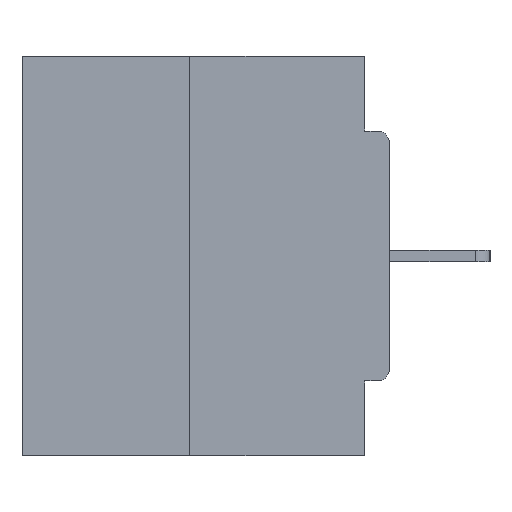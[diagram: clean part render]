
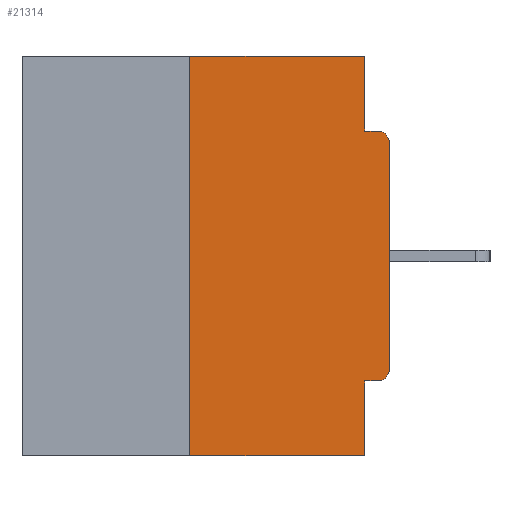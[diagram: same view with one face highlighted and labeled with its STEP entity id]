
A CAD part, left-side view. The second image highlights one B-rep face of the part: STEP entity #21314.
In plain terms, the highlighted planar face has unit normal (-1, 0, 0).
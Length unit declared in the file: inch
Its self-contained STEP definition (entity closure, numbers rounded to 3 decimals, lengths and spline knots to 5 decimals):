
#153 = VERTEX_POINT ( 'NONE', #30032 ) ;
#225 = LINE ( 'NONE', #2514, #6856 ) ;
#601 = EDGE_CURVE ( 'NONE', #12943, #153, #3066, .T. ) ;
#760 = EDGE_CURVE ( 'NONE', #32291, #30351, #11980, .T. ) ;
#1332 = CARTESIAN_POINT ( 'NONE',  ( 0., 0.031, -0.4065 ) ) ;
#1502 = CARTESIAN_POINT ( 'NONE',  ( 0., 0., -0.1085 ) ) ;
#1536 = LINE ( 'NONE', #28519, #22157 ) ;
#2011 = FACE_OUTER_BOUND ( 'NONE', #24314, .T. ) ;
#2514 = CARTESIAN_POINT ( 'NONE',  ( 0., 0., -0.4065 ) ) ;
#3066 = CIRCLE ( 'NONE', #21345, 0.015 ) ;
#3500 = VECTOR ( 'NONE', #28413, 39.37008 ) ;
#4495 = VERTEX_POINT ( 'NONE', #10970 ) ;
#4533 = EDGE_CURVE ( 'NONE', #22779, #26805, #20904, .T. ) ;
#5736 = VERTEX_POINT ( 'NONE', #13453 ) ;
#5785 = EDGE_CURVE ( 'NONE', #18133, #153, #11487, .T. ) ;
#6716 = EDGE_CURVE ( 'NONE', #5736, #18133, #19174, .T. ) ;
#6856 = VECTOR ( 'NONE', #17406, 39.37008 ) ;
#6939 = VECTOR ( 'NONE', #8908, 39.37008 ) ;
#7531 = CARTESIAN_POINT ( 'NONE',  ( 0., 0.031, -0.5 ) ) ;
#7620 = CARTESIAN_POINT ( 'NONE',  ( 0., 0.015, -0.1085 ) ) ;
#8199 = DIRECTION ( 'NONE',  ( 0., -1., 0. ) ) ;
#8374 = CARTESIAN_POINT ( 'NONE',  ( 0., 0.46, 0. ) ) ;
#8590 = AXIS2_PLACEMENT_3D ( 'NONE', #9398, #31938, #19516 ) ;
#8902 = DIRECTION ( 'NONE',  ( 0., -1., 0. ) ) ;
#8908 = DIRECTION ( 'NONE',  ( 0., 0., -1. ) ) ;
#9398 = CARTESIAN_POINT ( 'NONE',  ( 0., 0.46, 0. ) ) ;
#10970 = CARTESIAN_POINT ( 'NONE',  ( 0., 0.25, 0. ) ) ;
#11415 = VERTEX_POINT ( 'NONE', #11578 ) ;
#11487 = LINE ( 'NONE', #13925, #14600 ) ;
#11578 = CARTESIAN_POINT ( 'NONE',  ( 0., 0.25, -0.5 ) ) ;
#11980 = CIRCLE ( 'NONE', #13555, 0.015 ) ;
#12379 = DIRECTION ( 'NONE',  ( 0., 0., -1. ) ) ;
#12943 = VERTEX_POINT ( 'NONE', #1502 ) ;
#13190 = CARTESIAN_POINT ( 'NONE',  ( 0., 0., -0.3915 ) ) ;
#13239 = ORIENTED_EDGE ( 'NONE', *, *, #17939, .T. ) ;
#13453 = CARTESIAN_POINT ( 'NONE',  ( 0., 0.031, 0. ) ) ;
#13555 = AXIS2_PLACEMENT_3D ( 'NONE', #30490, #30153, #25245 ) ;
#13925 = CARTESIAN_POINT ( 'NONE',  ( 0., 0., -0.0935 ) ) ;
#14172 = ORIENTED_EDGE ( 'NONE', *, *, #6716, .F. ) ;
#14600 = VECTOR ( 'NONE', #23561, 39.37008 ) ;
#14655 = ORIENTED_EDGE ( 'NONE', *, *, #4533, .F. ) ;
#15375 = VECTOR ( 'NONE', #8199, 39.37008 ) ;
#15413 = VECTOR ( 'NONE', #24754, 39.37008 ) ;
#16392 = CARTESIAN_POINT ( 'NONE',  ( 0., 0.46, -0.5 ) ) ;
#16604 = EDGE_CURVE ( 'NONE', #32291, #22779, #225, .T. ) ;
#17406 = DIRECTION ( 'NONE',  ( 0., 1., 0. ) ) ;
#17939 = EDGE_CURVE ( 'NONE', #11415, #26805, #28186, .T. ) ;
#18133 = VERTEX_POINT ( 'NONE', #24721 ) ;
#18599 = CARTESIAN_POINT ( 'NONE',  ( 0., 0.031, -0.5 ) ) ;
#19174 = LINE ( 'NONE', #31441, #6939 ) ;
#19192 = DIRECTION ( 'NONE',  ( 0., 0., 1. ) ) ;
#19516 = DIRECTION ( 'NONE',  ( 0., 0., -1. ) ) ;
#19875 = DIRECTION ( 'NONE',  ( -1., 0., 0. ) ) ;
#20102 = EDGE_CURVE ( 'NONE', #4495, #5736, #27802, .T. ) ;
#20313 = ORIENTED_EDGE ( 'NONE', *, *, #16604, .F. ) ;
#20904 = LINE ( 'NONE', #18599, #3500 ) ;
#21314 = ADVANCED_FACE ( 'NONE', ( #2011 ), #21979, .F. ) ;
#21345 = AXIS2_PLACEMENT_3D ( 'NONE', #7620, #19875, #12379 ) ;
#21979 = PLANE ( 'NONE',  #8590 ) ;
#22157 = VECTOR ( 'NONE', #19192, 39.37008 ) ;
#22311 = LINE ( 'NONE', #31781, #15413 ) ;
#22345 = ORIENTED_EDGE ( 'NONE', *, *, #601, .T. ) ;
#22779 = VERTEX_POINT ( 'NONE', #1332 ) ;
#23561 = DIRECTION ( 'NONE',  ( 0., -1., 0. ) ) ;
#24314 = EDGE_LOOP ( 'NONE', ( #25982, #26920, #13239, #14655, #20313, #29840, #26096, #22345, #26098, #14172 ) ) ;
#24721 = CARTESIAN_POINT ( 'NONE',  ( 0., 0.031, -0.0935 ) ) ;
#24754 = DIRECTION ( 'NONE',  ( 0., 0., 1. ) ) ;
#25245 = DIRECTION ( 'NONE',  ( 0., 0., -1. ) ) ;
#25982 = ORIENTED_EDGE ( 'NONE', *, *, #20102, .F. ) ;
#26096 = ORIENTED_EDGE ( 'NONE', *, *, #27653, .T. ) ;
#26098 = ORIENTED_EDGE ( 'NONE', *, *, #5785, .F. ) ;
#26805 = VERTEX_POINT ( 'NONE', #7531 ) ;
#26920 = ORIENTED_EDGE ( 'NONE', *, *, #28961, .F. ) ;
#27653 = EDGE_CURVE ( 'NONE', #30351, #12943, #1536, .T. ) ;
#27780 = VECTOR ( 'NONE', #8902, 39.37008 ) ;
#27802 = LINE ( 'NONE', #8374, #15375 ) ;
#28186 = LINE ( 'NONE', #16392, #27780 ) ;
#28413 = DIRECTION ( 'NONE',  ( 0., 0., -1. ) ) ;
#28519 = CARTESIAN_POINT ( 'NONE',  ( 0., 0., 0. ) ) ;
#28961 = EDGE_CURVE ( 'NONE', #11415, #4495, #22311, .T. ) ;
#29065 = CARTESIAN_POINT ( 'NONE',  ( 0., 0.015, -0.4065 ) ) ;
#29840 = ORIENTED_EDGE ( 'NONE', *, *, #760, .T. ) ;
#30032 = CARTESIAN_POINT ( 'NONE',  ( 0., 0.015, -0.0935 ) ) ;
#30153 = DIRECTION ( 'NONE',  ( -1., 0., 0. ) ) ;
#30351 = VERTEX_POINT ( 'NONE', #13190 ) ;
#30490 = CARTESIAN_POINT ( 'NONE',  ( 0., 0.015, -0.3915 ) ) ;
#31441 = CARTESIAN_POINT ( 'NONE',  ( 0., 0.031, 0. ) ) ;
#31781 = CARTESIAN_POINT ( 'NONE',  ( 0., 0.25, 0. ) ) ;
#31938 = DIRECTION ( 'NONE',  ( 1., 0., 0. ) ) ;
#32291 = VERTEX_POINT ( 'NONE', #29065 ) ;
